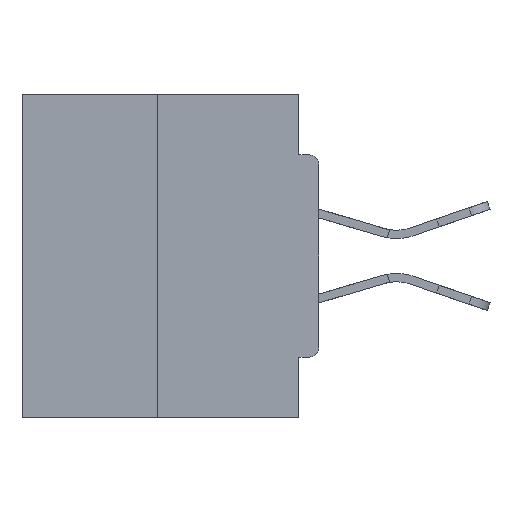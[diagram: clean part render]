
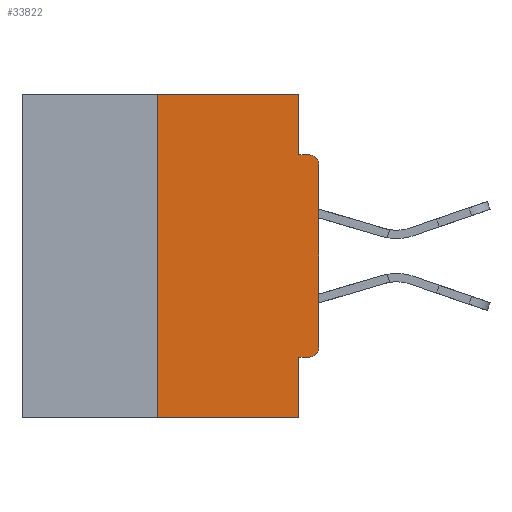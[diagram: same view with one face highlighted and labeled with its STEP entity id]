
A CAD part, left-side view. The second image highlights one B-rep face of the part: STEP entity #33822.
In plain terms, the highlighted planar face has unit normal (-1, 0, 0).
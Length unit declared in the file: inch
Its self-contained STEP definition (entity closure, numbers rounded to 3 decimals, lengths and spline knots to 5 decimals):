
#168 = LINE ( 'NONE', #17499, #40547 ) ;
#246 = DIRECTION ( 'NONE',  ( 0., -1., 0. ) ) ;
#532 = LINE ( 'NONE', #22328, #6056 ) ;
#611 = AXIS2_PLACEMENT_3D ( 'NONE', #34033, #14973, #8651 ) ;
#1195 = EDGE_CURVE ( 'NONE', #13216, #30377, #10286, .T. ) ;
#1764 = VECTOR ( 'NONE', #8053, 39.37008 ) ;
#1903 = CARTESIAN_POINT ( 'NONE',  ( 0., 0., -0.4065 ) ) ;
#2317 = ORIENTED_EDGE ( 'NONE', *, *, #2646, .F. ) ;
#2402 = VERTEX_POINT ( 'NONE', #20084 ) ;
#2646 = EDGE_CURVE ( 'NONE', #30377, #33881, #22710, .T. ) ;
#3737 = ORIENTED_EDGE ( 'NONE', *, *, #1195, .F. ) ;
#4355 = PLANE ( 'NONE',  #14086 ) ;
#4722 = VECTOR ( 'NONE', #37562, 39.37008 ) ;
#5164 = VERTEX_POINT ( 'NONE', #6235 ) ;
#5679 = CARTESIAN_POINT ( 'NONE',  ( 0., 0.031, 0. ) ) ;
#5708 = DIRECTION ( 'NONE',  ( 0., 0., -1. ) ) ;
#5814 = VERTEX_POINT ( 'NONE', #28609 ) ;
#6056 = VECTOR ( 'NONE', #246, 39.37008 ) ;
#6235 = CARTESIAN_POINT ( 'NONE',  ( 0., 0.25, -0.5 ) ) ;
#6383 = CARTESIAN_POINT ( 'NONE',  ( 0., 0., 0. ) ) ;
#6517 = CIRCLE ( 'NONE', #20693, 0.015 ) ;
#7935 = CARTESIAN_POINT ( 'NONE',  ( 0., 0.015, -0.4065 ) ) ;
#8053 = DIRECTION ( 'NONE',  ( 0., 1., 0. ) ) ;
#8651 = DIRECTION ( 'NONE',  ( 0., 0., -1. ) ) ;
#8713 = CARTESIAN_POINT ( 'NONE',  ( 0., 0.031, -0.4065 ) ) ;
#9914 = CARTESIAN_POINT ( 'NONE',  ( 0., 0., -0.3915 ) ) ;
#10184 = VECTOR ( 'NONE', #28926, 39.37008 ) ;
#10286 = LINE ( 'NONE', #1903, #1764 ) ;
#11192 = LINE ( 'NONE', #19027, #10184 ) ;
#12387 = ORIENTED_EDGE ( 'NONE', *, *, #18494, .F. ) ;
#12391 = EDGE_CURVE ( 'NONE', #2402, #12667, #25718, .T. ) ;
#12667 = VERTEX_POINT ( 'NONE', #30310 ) ;
#12847 = DIRECTION ( 'NONE',  ( 0., 0., 1. ) ) ;
#12959 = EDGE_LOOP ( 'NONE', ( #27840, #38766, #25774, #2317, #3737, #21599, #23616, #22807, #26674, #12387 ) ) ;
#13216 = VERTEX_POINT ( 'NONE', #7935 ) ;
#13750 = LINE ( 'NONE', #5679, #4722 ) ;
#13764 = DIRECTION ( 'NONE',  ( 0., 0., 1. ) ) ;
#14086 = AXIS2_PLACEMENT_3D ( 'NONE', #33258, #16948, #14171 ) ;
#14171 = DIRECTION ( 'NONE',  ( 0., 0., -1. ) ) ;
#14548 = CARTESIAN_POINT ( 'NONE',  ( 0., 0.015, -0.1085 ) ) ;
#14871 = EDGE_CURVE ( 'NONE', #25670, #20739, #6517, .T. ) ;
#14973 = DIRECTION ( 'NONE',  ( -1., 0., 0. ) ) ;
#15111 = EDGE_CURVE ( 'NONE', #13216, #37937, #22962, .T. ) ;
#15718 = VECTOR ( 'NONE', #5708, 39.37008 ) ;
#16948 = DIRECTION ( 'NONE',  ( 1., 0., 0. ) ) ;
#17499 = CARTESIAN_POINT ( 'NONE',  ( 0., 0.25, 0. ) ) ;
#18494 = EDGE_CURVE ( 'NONE', #12667, #5814, #13750, .T. ) ;
#19027 = CARTESIAN_POINT ( 'NONE',  ( 0., 0., -0.0935 ) ) ;
#20084 = CARTESIAN_POINT ( 'NONE',  ( 0., 0.25, 0. ) ) ;
#20190 = CARTESIAN_POINT ( 'NONE',  ( 0., 0.015, -0.0935 ) ) ;
#20670 = VECTOR ( 'NONE', #12847, 39.37008 ) ;
#20693 = AXIS2_PLACEMENT_3D ( 'NONE', #14548, #30558, #36793 ) ;
#20739 = VERTEX_POINT ( 'NONE', #20190 ) ;
#21599 = ORIENTED_EDGE ( 'NONE', *, *, #15111, .T. ) ;
#22328 = CARTESIAN_POINT ( 'NONE',  ( 0., 0.46, -0.5 ) ) ;
#22667 = FACE_OUTER_BOUND ( 'NONE', #12959, .T. ) ;
#22710 = LINE ( 'NONE', #24805, #15718 ) ;
#22807 = ORIENTED_EDGE ( 'NONE', *, *, #14871, .T. ) ;
#22962 = CIRCLE ( 'NONE', #611, 0.015 ) ;
#23616 = ORIENTED_EDGE ( 'NONE', *, *, #32718, .T. ) ;
#23768 = CARTESIAN_POINT ( 'NONE',  ( 0., 0.031, -0.5 ) ) ;
#24805 = CARTESIAN_POINT ( 'NONE',  ( 0., 0.031, -0.5 ) ) ;
#25670 = VERTEX_POINT ( 'NONE', #27922 ) ;
#25718 = LINE ( 'NONE', #27990, #26690 ) ;
#25774 = ORIENTED_EDGE ( 'NONE', *, *, #39933, .T. ) ;
#26674 = ORIENTED_EDGE ( 'NONE', *, *, #38725, .F. ) ;
#26690 = VECTOR ( 'NONE', #30633, 39.37008 ) ;
#27840 = ORIENTED_EDGE ( 'NONE', *, *, #12391, .F. ) ;
#27922 = CARTESIAN_POINT ( 'NONE',  ( 0., 0., -0.1085 ) ) ;
#27990 = CARTESIAN_POINT ( 'NONE',  ( 0., 0.46, 0. ) ) ;
#28609 = CARTESIAN_POINT ( 'NONE',  ( 0., 0.031, -0.0935 ) ) ;
#28926 = DIRECTION ( 'NONE',  ( 0., -1., 0. ) ) ;
#30310 = CARTESIAN_POINT ( 'NONE',  ( 0., 0.031, 0. ) ) ;
#30377 = VERTEX_POINT ( 'NONE', #8713 ) ;
#30558 = DIRECTION ( 'NONE',  ( -1., 0., 0. ) ) ;
#30633 = DIRECTION ( 'NONE',  ( 0., -1., 0. ) ) ;
#32718 = EDGE_CURVE ( 'NONE', #37937, #25670, #38583, .T. ) ;
#33258 = CARTESIAN_POINT ( 'NONE',  ( 0., 0.46, 0. ) ) ;
#33807 = EDGE_CURVE ( 'NONE', #5164, #2402, #168, .T. ) ;
#33822 = ADVANCED_FACE ( 'NONE', ( #22667 ), #4355, .F. ) ;
#33881 = VERTEX_POINT ( 'NONE', #23768 ) ;
#34033 = CARTESIAN_POINT ( 'NONE',  ( 0., 0.015, -0.3915 ) ) ;
#36793 = DIRECTION ( 'NONE',  ( 0., 0., -1. ) ) ;
#37562 = DIRECTION ( 'NONE',  ( 0., 0., -1. ) ) ;
#37937 = VERTEX_POINT ( 'NONE', #9914 ) ;
#38583 = LINE ( 'NONE', #6383, #20670 ) ;
#38725 = EDGE_CURVE ( 'NONE', #5814, #20739, #11192, .T. ) ;
#38766 = ORIENTED_EDGE ( 'NONE', *, *, #33807, .F. ) ;
#39933 = EDGE_CURVE ( 'NONE', #5164, #33881, #532, .T. ) ;
#40547 = VECTOR ( 'NONE', #13764, 39.37008 ) ;
